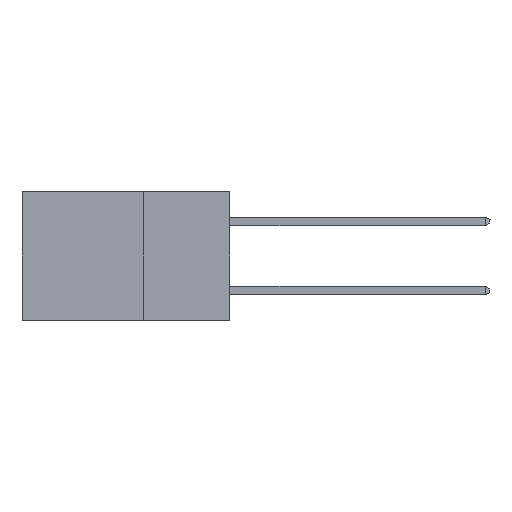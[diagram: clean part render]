
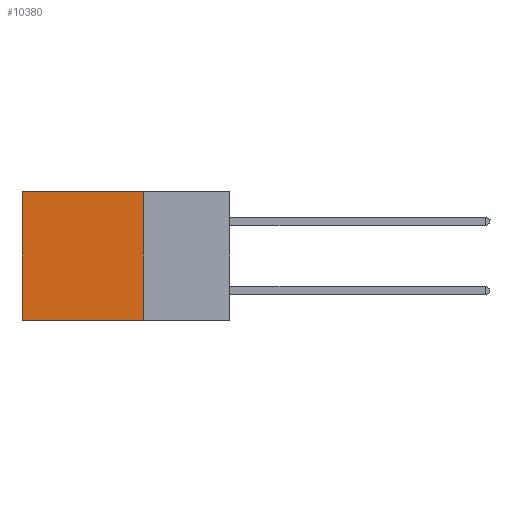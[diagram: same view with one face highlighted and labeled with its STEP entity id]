
A CAD part, left-side view. The second image highlights one B-rep face of the part: STEP entity #10380.
In plain terms, the highlighted planar face has unit normal (-1, 0, 0).
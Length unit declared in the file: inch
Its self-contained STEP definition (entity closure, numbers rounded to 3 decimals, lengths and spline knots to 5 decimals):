
#288 = DIRECTION ( 'NONE',  ( 1., 0., 0. ) ) ;
#450 = PLANE ( 'NONE',  #2552 ) ;
#1321 = CARTESIAN_POINT ( 'NONE',  ( 0.298, 0.25, 0. ) ) ;
#1512 = CARTESIAN_POINT ( 'NONE',  ( 0.298, 0.25, 0. ) ) ;
#2039 = EDGE_LOOP ( 'NONE', ( #4811, #2923, #10856, #5526 ) ) ;
#2552 = AXIS2_PLACEMENT_3D ( 'NONE', #1321, #288, #5400 ) ;
#2797 = DIRECTION ( 'NONE',  ( 0., 1., 0. ) ) ;
#2923 = ORIENTED_EDGE ( 'NONE', *, *, #5302, .F. ) ;
#2939 = LINE ( 'NONE', #7998, #10257 ) ;
#4610 = CARTESIAN_POINT ( 'NONE',  ( 0.298, 0.6, 0. ) ) ;
#4811 = ORIENTED_EDGE ( 'NONE', *, *, #10895, .T. ) ;
#4853 = VERTEX_POINT ( 'NONE', #6035 ) ;
#5302 = EDGE_CURVE ( 'NONE', #10216, #4853, #7235, .T. ) ;
#5332 = DIRECTION ( 'NONE',  ( 0., 0., -1. ) ) ;
#5400 = DIRECTION ( 'NONE',  ( 0., 0., -1. ) ) ;
#5526 = ORIENTED_EDGE ( 'NONE', *, *, #8665, .T. ) ;
#5775 = VERTEX_POINT ( 'NONE', #4610 ) ;
#6035 = CARTESIAN_POINT ( 'NONE',  ( 0.298, 0.6, -0.37 ) ) ;
#6813 = CARTESIAN_POINT ( 'NONE',  ( 0.298, 0.25, -0.37 ) ) ;
#7235 = LINE ( 'NONE', #6813, #9572 ) ;
#7576 = LINE ( 'NONE', #12115, #8200 ) ;
#7998 = CARTESIAN_POINT ( 'NONE',  ( 0.298, 0.25, 0. ) ) ;
#8200 = VECTOR ( 'NONE', #10225, 39.37008 ) ;
#8665 = EDGE_CURVE ( 'NONE', #10473, #5775, #2939, .T. ) ;
#8700 = VECTOR ( 'NONE', #5332, 39.37008 ) ;
#9087 = CARTESIAN_POINT ( 'NONE',  ( 0.298, 0.25, -0.37 ) ) ;
#9250 = CARTESIAN_POINT ( 'NONE',  ( 0.298, 0.25, 0. ) ) ;
#9279 = DIRECTION ( 'NONE',  ( 0., 1., 0. ) ) ;
#9572 = VECTOR ( 'NONE', #2797, 39.37008 ) ;
#9776 = FACE_OUTER_BOUND ( 'NONE', #2039, .T. ) ;
#9845 = EDGE_CURVE ( 'NONE', #10473, #10216, #11183, .T. ) ;
#10216 = VERTEX_POINT ( 'NONE', #9087 ) ;
#10225 = DIRECTION ( 'NONE',  ( 0., 0., -1. ) ) ;
#10257 = VECTOR ( 'NONE', #9279, 39.37008 ) ;
#10380 = ADVANCED_FACE ( 'NONE', ( #9776 ), #450, .F. ) ;
#10473 = VERTEX_POINT ( 'NONE', #1512 ) ;
#10856 = ORIENTED_EDGE ( 'NONE', *, *, #9845, .F. ) ;
#10895 = EDGE_CURVE ( 'NONE', #5775, #4853, #7576, .T. ) ;
#11183 = LINE ( 'NONE', #9250, #8700 ) ;
#12115 = CARTESIAN_POINT ( 'NONE',  ( 0.298, 0.6, 0. ) ) ;
